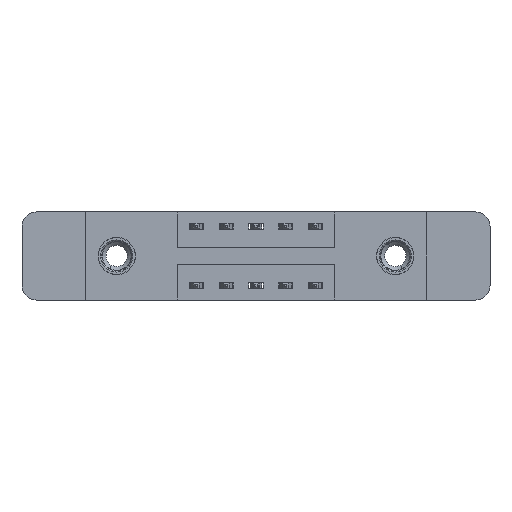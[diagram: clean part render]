
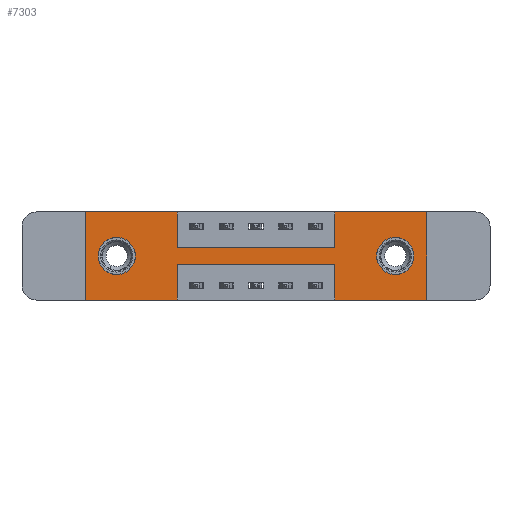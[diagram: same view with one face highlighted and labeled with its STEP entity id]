
A CAD part, front view. The second image highlights one B-rep face of the part: STEP entity #7303.
In plain terms, the highlighted planar face has unit normal (0, -1, 0).
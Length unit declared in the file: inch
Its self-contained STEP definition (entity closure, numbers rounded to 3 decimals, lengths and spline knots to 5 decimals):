
#11 = VERTEX_POINT ( 'NONE', #10759 ) ;
#128 = CARTESIAN_POINT ( 'NONE',  ( 1.0475, 0., -0.37 ) ) ;
#448 = CARTESIAN_POINT ( 'NONE',  ( 0.1325, 0., -0.263 ) ) ;
#475 = ORIENTED_EDGE ( 'NONE', *, *, #708, .F. ) ;
#539 = ORIENTED_EDGE ( 'NONE', *, *, #13348, .F. ) ;
#708 = EDGE_CURVE ( 'NONE', #11, #6641, #2877, .T. ) ;
#851 = VERTEX_POINT ( 'NONE', #1857 ) ;
#1200 = EDGE_CURVE ( 'NONE', #6293, #7450, #5075, .T. ) ;
#1296 = PLANE ( 'NONE',  #11825 ) ;
#1389 = DIRECTION ( 'NONE',  ( 0., 0., -1. ) ) ;
#1419 = EDGE_CURVE ( 'NONE', #4798, #10071, #3501, .T. ) ;
#1454 = VERTEX_POINT ( 'NONE', #2375 ) ;
#1583 = DIRECTION ( 'NONE',  ( 0., 1., 0. ) ) ;
#1836 = VECTOR ( 'NONE', #8248, 39.37008 ) ;
#1857 = CARTESIAN_POINT ( 'NONE',  ( 0.1325, 0., -0.107 ) ) ;
#1937 = VERTEX_POINT ( 'NONE', #3449 ) ;
#1964 = VERTEX_POINT ( 'NONE', #6632 ) ;
#2311 = DIRECTION ( 'NONE',  ( 1., 0., 0. ) ) ;
#2321 = DIRECTION ( 'NONE',  ( 0., 1., 0. ) ) ;
#2375 = CARTESIAN_POINT ( 'NONE',  ( 1.435, 0., -0.37 ) ) ;
#2408 = EDGE_LOOP ( 'NONE', ( #3857, #9469, #539, #11587, #10393, #4440, #4115, #11280, #7556, #2944, #8509, #475 ) ) ;
#2463 = CARTESIAN_POINT ( 'NONE',  ( 0., 0., 0. ) ) ;
#2571 = EDGE_CURVE ( 'NONE', #11780, #11, #7649, .T. ) ;
#2578 = DIRECTION ( 'NONE',  ( -1., 0., 0. ) ) ;
#2639 = DIRECTION ( 'NONE',  ( -1., 0., 0. ) ) ;
#2647 = VECTOR ( 'NONE', #2639, 39.37008 ) ;
#2666 = FACE_OUTER_BOUND ( 'NONE', #2408, .T. ) ;
#2683 = EDGE_CURVE ( 'NONE', #1964, #10403, #5381, .T. ) ;
#2743 = VERTEX_POINT ( 'NONE', #7308 ) ;
#2858 = DIRECTION ( 'NONE',  ( 0., 0., -1. ) ) ;
#2877 = LINE ( 'NONE', #11743, #12926 ) ;
#2928 = VERTEX_POINT ( 'NONE', #448 ) ;
#2944 = ORIENTED_EDGE ( 'NONE', *, *, #5032, .F. ) ;
#3282 = CARTESIAN_POINT ( 'NONE',  ( 1.435, 0., 0. ) ) ;
#3345 = DIRECTION ( 'NONE',  ( 0., -1., 0. ) ) ;
#3407 = DIRECTION ( 'NONE',  ( 0., 0., -1. ) ) ;
#3433 = EDGE_CURVE ( 'NONE', #2743, #1964, #5338, .T. ) ;
#3449 = CARTESIAN_POINT ( 'NONE',  ( 0., 0., 0. ) ) ;
#3501 = CIRCLE ( 'NONE', #9666, 0.078 ) ;
#3832 = EDGE_LOOP ( 'NONE', ( #4371, #9314 ) ) ;
#3840 = DIRECTION ( 'NONE',  ( 0., 0., 1. ) ) ;
#3857 = ORIENTED_EDGE ( 'NONE', *, *, #2571, .F. ) ;
#3975 = CARTESIAN_POINT ( 'NONE',  ( 0., 0., -0.37 ) ) ;
#3980 = DIRECTION ( 'NONE',  ( 0., 0., -1. ) ) ;
#4115 = ORIENTED_EDGE ( 'NONE', *, *, #7821, .F. ) ;
#4371 = ORIENTED_EDGE ( 'NONE', *, *, #12924, .T. ) ;
#4440 = ORIENTED_EDGE ( 'NONE', *, *, #1200, .F. ) ;
#4552 = DIRECTION ( 'NONE',  ( 0., 0., -1. ) ) ;
#4798 = VERTEX_POINT ( 'NONE', #5464 ) ;
#4901 = DIRECTION ( 'NONE',  ( 0., 1., 0. ) ) ;
#4989 = EDGE_CURVE ( 'NONE', #1454, #13100, #9294, .T. ) ;
#5032 = EDGE_CURVE ( 'NONE', #1937, #2743, #5755, .T. ) ;
#5075 = LINE ( 'NONE', #12348, #1836 ) ;
#5154 = CARTESIAN_POINT ( 'NONE',  ( 1.0475, 0., 0. ) ) ;
#5338 = LINE ( 'NONE', #9218, #13472 ) ;
#5381 = LINE ( 'NONE', #9037, #12993 ) ;
#5432 = CIRCLE ( 'NONE', #6937, 0.078 ) ;
#5464 = CARTESIAN_POINT ( 'NONE',  ( 1.3025, 0., -0.263 ) ) ;
#5483 = CARTESIAN_POINT ( 'NONE',  ( 1.435, 0., 0. ) ) ;
#5755 = LINE ( 'NONE', #2463, #10603 ) ;
#5965 = VECTOR ( 'NONE', #1389, 39.37008 ) ;
#6293 = VERTEX_POINT ( 'NONE', #5154 ) ;
#6632 = CARTESIAN_POINT ( 'NONE',  ( 0.3875, 0., -0.15 ) ) ;
#6641 = VERTEX_POINT ( 'NONE', #12014 ) ;
#6862 = CARTESIAN_POINT ( 'NONE',  ( 0.1325, 0., -0.185 ) ) ;
#6937 = AXIS2_PLACEMENT_3D ( 'NONE', #6862, #1583, #3840 ) ;
#7029 = CARTESIAN_POINT ( 'NONE',  ( 1.3025, 0., -0.185 ) ) ;
#7255 = DIRECTION ( 'NONE',  ( 0., 1., 0. ) ) ;
#7303 = ADVANCED_FACE ( 'NONE', ( #7835, #8627, #2666 ), #1296, .T. ) ;
#7307 = EDGE_CURVE ( 'NONE', #11965, #11780, #11062, .T. ) ;
#7308 = CARTESIAN_POINT ( 'NONE',  ( 0.3875, 0., 0. ) ) ;
#7450 = VERTEX_POINT ( 'NONE', #3282 ) ;
#7516 = AXIS2_PLACEMENT_3D ( 'NONE', #7029, #4901, #2858 ) ;
#7556 = ORIENTED_EDGE ( 'NONE', *, *, #3433, .F. ) ;
#7649 = LINE ( 'NONE', #7755, #8908 ) ;
#7755 = CARTESIAN_POINT ( 'NONE',  ( 0.3875, 0., -0.37 ) ) ;
#7821 = EDGE_CURVE ( 'NONE', #10403, #6293, #11238, .T. ) ;
#7831 = VECTOR ( 'NONE', #12085, 39.37008 ) ;
#7835 = FACE_BOUND ( 'NONE', #3832, .T. ) ;
#7856 = LINE ( 'NONE', #9891, #8335 ) ;
#7871 = VECTOR ( 'NONE', #10250, 39.37008 ) ;
#7884 = DIRECTION ( 'NONE',  ( 0., 0., 1. ) ) ;
#7897 = EDGE_CURVE ( 'NONE', #6641, #1937, #10387, .T. ) ;
#8238 = DIRECTION ( 'NONE',  ( 1., 0., 0. ) ) ;
#8248 = DIRECTION ( 'NONE',  ( 1., 0., 0. ) ) ;
#8266 = DIRECTION ( 'NONE',  ( 0., 0., 1. ) ) ;
#8335 = VECTOR ( 'NONE', #7884, 39.37008 ) ;
#8472 = CARTESIAN_POINT ( 'NONE',  ( 1.3025, 0., -0.185 ) ) ;
#8509 = ORIENTED_EDGE ( 'NONE', *, *, #7897, .F. ) ;
#8627 = FACE_BOUND ( 'NONE', #11692, .T. ) ;
#8714 = LINE ( 'NONE', #5483, #5965 ) ;
#8792 = DIRECTION ( 'NONE',  ( 0., 0., -1. ) ) ;
#8908 = VECTOR ( 'NONE', #8792, 39.37008 ) ;
#9011 = EDGE_CURVE ( 'NONE', #2928, #851, #12929, .T. ) ;
#9037 = CARTESIAN_POINT ( 'NONE',  ( 0.3875, 0., -0.15 ) ) ;
#9126 = DIRECTION ( 'NONE',  ( 0., 0., 1. ) ) ;
#9184 = AXIS2_PLACEMENT_3D ( 'NONE', #12249, #7255, #9126 ) ;
#9218 = CARTESIAN_POINT ( 'NONE',  ( 0.3875, 0., 0. ) ) ;
#9294 = LINE ( 'NONE', #3975, #7871 ) ;
#9314 = ORIENTED_EDGE ( 'NONE', *, *, #1419, .T. ) ;
#9469 = ORIENTED_EDGE ( 'NONE', *, *, #7307, .F. ) ;
#9483 = CARTESIAN_POINT ( 'NONE',  ( 0., 0., -0.37 ) ) ;
#9666 = AXIS2_PLACEMENT_3D ( 'NONE', #8472, #2321, #3407 ) ;
#9891 = CARTESIAN_POINT ( 'NONE',  ( 1.0475, 0., -0.37 ) ) ;
#10050 = VECTOR ( 'NONE', #8266, 39.37008 ) ;
#10071 = VERTEX_POINT ( 'NONE', #12093 ) ;
#10250 = DIRECTION ( 'NONE',  ( -1., 0., 0. ) ) ;
#10387 = LINE ( 'NONE', #11506, #10050 ) ;
#10393 = ORIENTED_EDGE ( 'NONE', *, *, #10854, .F. ) ;
#10403 = VERTEX_POINT ( 'NONE', #10739 ) ;
#10603 = VECTOR ( 'NONE', #2311, 39.37008 ) ;
#10739 = CARTESIAN_POINT ( 'NONE',  ( 1.0475, 0., -0.15 ) ) ;
#10759 = CARTESIAN_POINT ( 'NONE',  ( 0.3875, 0., -0.37 ) ) ;
#10854 = EDGE_CURVE ( 'NONE', #7450, #1454, #8714, .T. ) ;
#11062 = LINE ( 'NONE', #12953, #2647 ) ;
#11109 = CARTESIAN_POINT ( 'NONE',  ( 1.0475, 0., 0. ) ) ;
#11238 = LINE ( 'NONE', #11109, #7831 ) ;
#11280 = ORIENTED_EDGE ( 'NONE', *, *, #2683, .F. ) ;
#11506 = CARTESIAN_POINT ( 'NONE',  ( 0., 0., 0. ) ) ;
#11560 = ORIENTED_EDGE ( 'NONE', *, *, #13329, .T. ) ;
#11587 = ORIENTED_EDGE ( 'NONE', *, *, #4989, .F. ) ;
#11692 = EDGE_LOOP ( 'NONE', ( #11560, #12412 ) ) ;
#11743 = CARTESIAN_POINT ( 'NONE',  ( 0., 0., -0.37 ) ) ;
#11780 = VERTEX_POINT ( 'NONE', #11978 ) ;
#11825 = AXIS2_PLACEMENT_3D ( 'NONE', #9483, #3345, #4552 ) ;
#11965 = VERTEX_POINT ( 'NONE', #13409 ) ;
#11978 = CARTESIAN_POINT ( 'NONE',  ( 0.3875, 0., -0.22 ) ) ;
#12014 = CARTESIAN_POINT ( 'NONE',  ( 0., 0., -0.37 ) ) ;
#12085 = DIRECTION ( 'NONE',  ( 0., 0., 1. ) ) ;
#12093 = CARTESIAN_POINT ( 'NONE',  ( 1.3025, 0., -0.107 ) ) ;
#12249 = CARTESIAN_POINT ( 'NONE',  ( 0.1325, 0., -0.185 ) ) ;
#12348 = CARTESIAN_POINT ( 'NONE',  ( 0., 0., 0. ) ) ;
#12412 = ORIENTED_EDGE ( 'NONE', *, *, #9011, .T. ) ;
#12723 = CIRCLE ( 'NONE', #7516, 0.078 ) ;
#12924 = EDGE_CURVE ( 'NONE', #10071, #4798, #12723, .T. ) ;
#12926 = VECTOR ( 'NONE', #2578, 39.37008 ) ;
#12929 = CIRCLE ( 'NONE', #9184, 0.078 ) ;
#12953 = CARTESIAN_POINT ( 'NONE',  ( 0.3875, 0., -0.22 ) ) ;
#12993 = VECTOR ( 'NONE', #8238, 39.37008 ) ;
#13100 = VERTEX_POINT ( 'NONE', #128 ) ;
#13329 = EDGE_CURVE ( 'NONE', #851, #2928, #5432, .T. ) ;
#13348 = EDGE_CURVE ( 'NONE', #13100, #11965, #7856, .T. ) ;
#13409 = CARTESIAN_POINT ( 'NONE',  ( 1.0475, 0., -0.22 ) ) ;
#13472 = VECTOR ( 'NONE', #3980, 39.37008 ) ;
